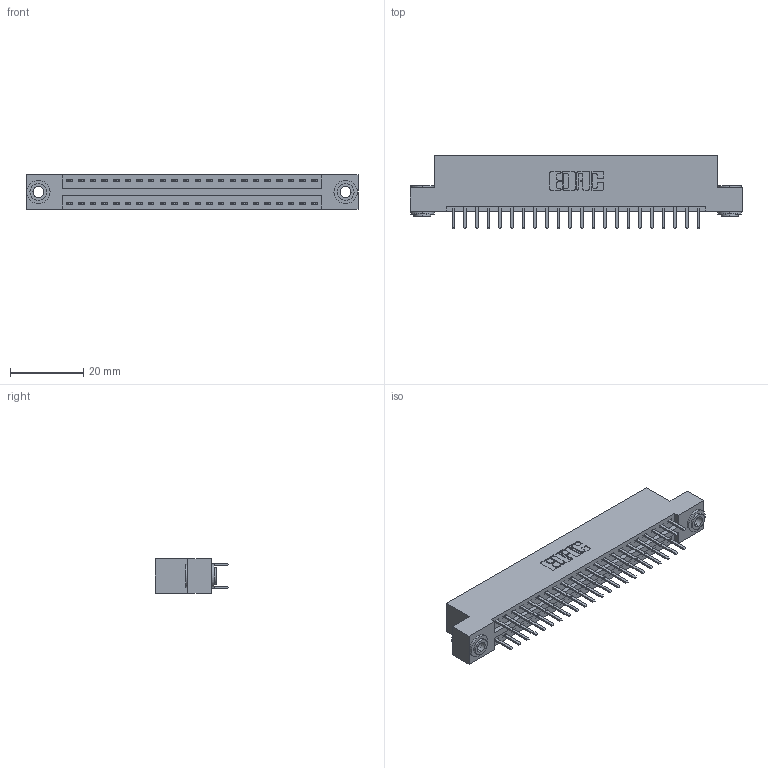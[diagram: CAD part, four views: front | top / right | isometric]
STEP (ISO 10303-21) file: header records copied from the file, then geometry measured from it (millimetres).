
FILE_DESCRIPTION (( 'STEP AP203' ), '1' );
FILE_NAME ('396-044-520-203.STEP', '2018-09-07T03:04:49', ( '' ), ( '' ), 'SwSTEP 2.0', 'SolidWorks 2016', '' );
FILE_SCHEMA (( 'CONFIG_CONTROL_DESIGN' ));
Length unit declared in the file: inch
Products named in the file (4): 346 Part_Flush Mounting Lugs - 0.156 Dia-TH; 345-292-001_345-293-120; 345-250-002_345-250-002-102; 396-044-520-203
Assembly tree (47 placements, depth 2):
  396-044-520-203
    346 Part_Flush Mounting Lugs - 0.156 Dia-TH
    345-292-001_345-293-120  x44
    345-250-002_345-250-002-102  x2
Bounding box: 90.42 x 20.02 x 9.4 mm (x, y, z)
Volume: 8662.2 mm3; surface area: 11761.3 mm2
Topology: 47 solids, 47 shells, 2624 faces, 7577 edges, 4930 vertices
Faces by surface type: plane 1714, cylinder 902, cone 8
Entity records: 17814 total; most frequent: CARTESIAN_POINT 2951, ORIENTED_EDGE 2866, DIRECTION 2671, EDGE_CURVE 1433, LINE 1185, VECTOR 1185, VERTEX_POINT 950, AXIS2_PLACEMENT_3D 743
